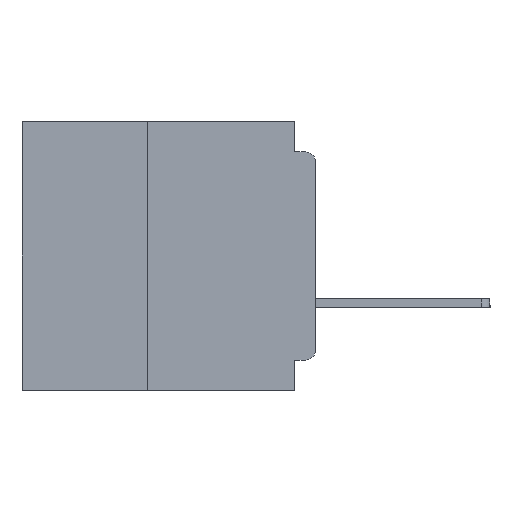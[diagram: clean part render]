
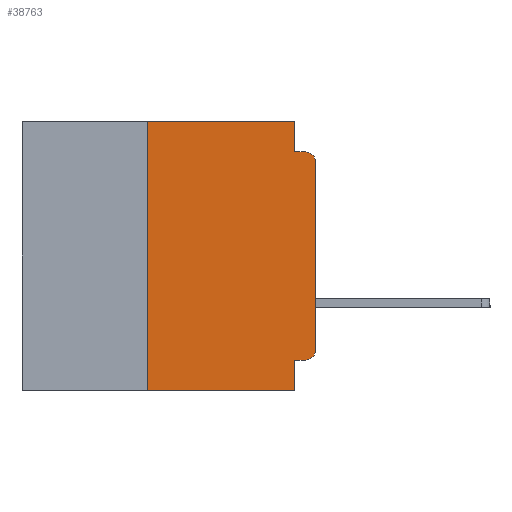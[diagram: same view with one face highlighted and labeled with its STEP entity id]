
A CAD part, left-side view. The second image highlights one B-rep face of the part: STEP entity #38763.
In plain terms, the highlighted planar face has unit normal (-1, 0, 0).
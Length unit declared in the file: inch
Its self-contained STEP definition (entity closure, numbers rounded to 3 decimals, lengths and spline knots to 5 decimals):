
#833 = CARTESIAN_POINT ( 'NONE',  ( 0., 0.031, -0.4 ) ) ;
#1275 = ORIENTED_EDGE ( 'NONE', *, *, #38735, .T. ) ;
#1495 = DIRECTION ( 'NONE',  ( -1., 0., 0. ) ) ;
#2254 = LINE ( 'NONE', #15361, #3402 ) ;
#2615 = CARTESIAN_POINT ( 'NONE',  ( 0., 0.031, -0.4 ) ) ;
#3402 = VECTOR ( 'NONE', #37266, 39.37008 ) ;
#3433 = VERTEX_POINT ( 'NONE', #26564 ) ;
#4640 = CARTESIAN_POINT ( 'NONE',  ( 0., 0.015, -0.355 ) ) ;
#5158 = FACE_OUTER_BOUND ( 'NONE', #7824, .T. ) ;
#5279 = ORIENTED_EDGE ( 'NONE', *, *, #20466, .F. ) ;
#6524 = VECTOR ( 'NONE', #44460, 39.37008 ) ;
#6601 = VERTEX_POINT ( 'NONE', #23794 ) ;
#6870 = VECTOR ( 'NONE', #8177, 39.37008 ) ;
#7015 = VECTOR ( 'NONE', #39408, 39.37008 ) ;
#7681 = LINE ( 'NONE', #37251, #6524 ) ;
#7824 = EDGE_LOOP ( 'NONE', ( #1275, #29989, #5279, #7896, #23535, #11905, #32336, #28544, #26964, #39403 ) ) ;
#7896 = ORIENTED_EDGE ( 'NONE', *, *, #28738, .F. ) ;
#8177 = DIRECTION ( 'NONE',  ( 0., 1., 0. ) ) ;
#8189 = CARTESIAN_POINT ( 'NONE',  ( 0., 0.25, -0.4 ) ) ;
#8547 = EDGE_CURVE ( 'NONE', #33265, #3433, #17773, .T. ) ;
#9180 = EDGE_CURVE ( 'NONE', #19043, #31508, #36606, .T. ) ;
#10169 = CARTESIAN_POINT ( 'NONE',  ( 0., 0., -0.06 ) ) ;
#10935 = CARTESIAN_POINT ( 'NONE',  ( 0., 0.437, 0. ) ) ;
#11197 = CARTESIAN_POINT ( 'NONE',  ( 0., 0.015, -0.045 ) ) ;
#11248 = DIRECTION ( 'NONE',  ( 0., 0., -1. ) ) ;
#11905 = ORIENTED_EDGE ( 'NONE', *, *, #8547, .F. ) ;
#13740 = DIRECTION ( 'NONE',  ( 0., 0., -1. ) ) ;
#14183 = CARTESIAN_POINT ( 'NONE',  ( 0., 0.015, -0.06 ) ) ;
#14598 = VERTEX_POINT ( 'NONE', #18244 ) ;
#15010 = VECTOR ( 'NONE', #29377, 39.37008 ) ;
#15361 = CARTESIAN_POINT ( 'NONE',  ( 0., 0., -0.045 ) ) ;
#15597 = CARTESIAN_POINT ( 'NONE',  ( 0., 0., -0.355 ) ) ;
#17773 = LINE ( 'NONE', #43355, #34932 ) ;
#17879 = DIRECTION ( 'NONE',  ( 0., 0., -1. ) ) ;
#18244 = CARTESIAN_POINT ( 'NONE',  ( 0., 0., -0.34 ) ) ;
#19043 = VERTEX_POINT ( 'NONE', #10169 ) ;
#20466 = EDGE_CURVE ( 'NONE', #22295, #31508, #2254, .T. ) ;
#21047 = CARTESIAN_POINT ( 'NONE',  ( 0., 0.031, 0. ) ) ;
#21893 = CARTESIAN_POINT ( 'NONE',  ( 0., 0.437, 0. ) ) ;
#22295 = VERTEX_POINT ( 'NONE', #37489 ) ;
#23005 = EDGE_CURVE ( 'NONE', #40174, #14598, #33084, .T. ) ;
#23535 = ORIENTED_EDGE ( 'NONE', *, *, #37399, .F. ) ;
#23554 = CARTESIAN_POINT ( 'NONE',  ( 0., 0.015, -0.34 ) ) ;
#23794 = CARTESIAN_POINT ( 'NONE',  ( 0., 0.031, -0.355 ) ) ;
#24043 = EDGE_CURVE ( 'NONE', #40174, #6601, #29871, .T. ) ;
#24912 = LINE ( 'NONE', #21893, #33448 ) ;
#25731 = CARTESIAN_POINT ( 'NONE',  ( 0., 0., 0. ) ) ;
#26097 = EDGE_CURVE ( 'NONE', #6601, #26394, #40523, .T. ) ;
#26394 = VERTEX_POINT ( 'NONE', #833 ) ;
#26564 = CARTESIAN_POINT ( 'NONE',  ( 0., 0.25, 0. ) ) ;
#26596 = LINE ( 'NONE', #35716, #7015 ) ;
#26964 = ORIENTED_EDGE ( 'NONE', *, *, #24043, .F. ) ;
#27211 = DIRECTION ( 'NONE',  ( 0., 0., -1. ) ) ;
#28275 = AXIS2_PLACEMENT_3D ( 'NONE', #14183, #39799, #17879 ) ;
#28544 = ORIENTED_EDGE ( 'NONE', *, *, #26097, .F. ) ;
#28738 = EDGE_CURVE ( 'NONE', #36042, #22295, #26596, .T. ) ;
#29377 = DIRECTION ( 'NONE',  ( 0., 0., 1. ) ) ;
#29871 = LINE ( 'NONE', #15597, #6870 ) ;
#29989 = ORIENTED_EDGE ( 'NONE', *, *, #9180, .T. ) ;
#31508 = VERTEX_POINT ( 'NONE', #11197 ) ;
#32336 = ORIENTED_EDGE ( 'NONE', *, *, #34456, .T. ) ;
#32881 = DIRECTION ( 'NONE',  ( 0., -1., 0. ) ) ;
#33084 = CIRCLE ( 'NONE', #46021, 0.015 ) ;
#33202 = DIRECTION ( 'NONE',  ( 1., 0., 0. ) ) ;
#33265 = VERTEX_POINT ( 'NONE', #8189 ) ;
#33448 = VECTOR ( 'NONE', #32881, 39.37008 ) ;
#34456 = EDGE_CURVE ( 'NONE', #33265, #26394, #7681, .T. ) ;
#34932 = VECTOR ( 'NONE', #36170, 39.37008 ) ;
#35716 = CARTESIAN_POINT ( 'NONE',  ( 0., 0.031, 0. ) ) ;
#36042 = VERTEX_POINT ( 'NONE', #21047 ) ;
#36170 = DIRECTION ( 'NONE',  ( 0., 0., 1. ) ) ;
#36606 = CIRCLE ( 'NONE', #28275, 0.015 ) ;
#37251 = CARTESIAN_POINT ( 'NONE',  ( 0., 0.437, -0.4 ) ) ;
#37266 = DIRECTION ( 'NONE',  ( 0., -1., 0. ) ) ;
#37399 = EDGE_CURVE ( 'NONE', #3433, #36042, #24912, .T. ) ;
#37489 = CARTESIAN_POINT ( 'NONE',  ( 0., 0.031, -0.045 ) ) ;
#38735 = EDGE_CURVE ( 'NONE', #14598, #19043, #44212, .T. ) ;
#38763 = ADVANCED_FACE ( 'NONE', ( #5158 ), #44086, .F. ) ;
#39374 = VECTOR ( 'NONE', #13740, 39.37008 ) ;
#39403 = ORIENTED_EDGE ( 'NONE', *, *, #23005, .T. ) ;
#39408 = DIRECTION ( 'NONE',  ( 0., 0., -1. ) ) ;
#39799 = DIRECTION ( 'NONE',  ( -1., 0., 0. ) ) ;
#39810 = AXIS2_PLACEMENT_3D ( 'NONE', #10935, #33202, #11248 ) ;
#40174 = VERTEX_POINT ( 'NONE', #4640 ) ;
#40523 = LINE ( 'NONE', #2615, #39374 ) ;
#43355 = CARTESIAN_POINT ( 'NONE',  ( 0., 0.25, -0.4 ) ) ;
#44086 = PLANE ( 'NONE',  #39810 ) ;
#44212 = LINE ( 'NONE', #25731, #15010 ) ;
#44460 = DIRECTION ( 'NONE',  ( 0., -1., 0. ) ) ;
#46021 = AXIS2_PLACEMENT_3D ( 'NONE', #23554, #1495, #27211 ) ;
